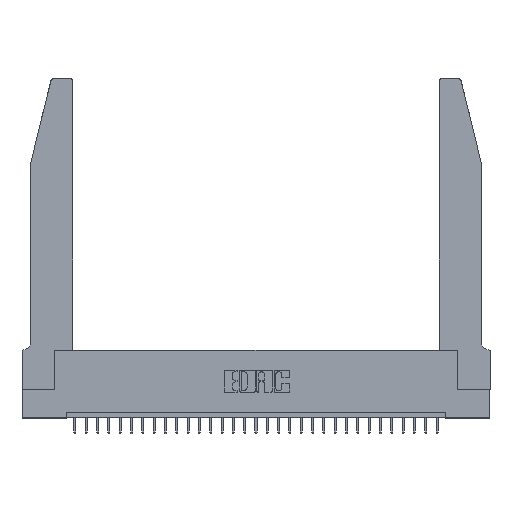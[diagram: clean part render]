
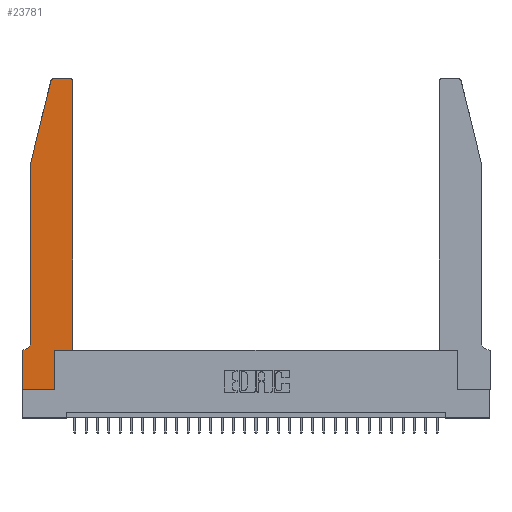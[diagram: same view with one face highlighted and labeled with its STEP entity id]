
A CAD part, top view. The second image highlights one B-rep face of the part: STEP entity #23781.
In plain terms, the highlighted planar face has unit normal (0, 0, 1).
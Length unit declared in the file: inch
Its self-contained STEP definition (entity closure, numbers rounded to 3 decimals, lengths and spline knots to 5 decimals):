
#175 = CARTESIAN_POINT ( 'NONE',  ( 0., 0., 0.37 ) ) ;
#258 = CARTESIAN_POINT ( 'NONE',  ( 0.0055, 0.42, 0.37 ) ) ;
#1079 = VECTOR ( 'NONE', #3744, 39.37008 ) ;
#1533 = VECTOR ( 'NONE', #15672, 39.37008 ) ;
#2079 = EDGE_CURVE ( 'NONE', #27720, #7704, #17153, .T. ) ;
#2528 = CARTESIAN_POINT ( 'NONE',  ( 0.0755, 0.35, 0.37 ) ) ;
#3563 = LINE ( 'NONE', #13246, #11403 ) ;
#3694 = EDGE_CURVE ( 'NONE', #10968, #28322, #28476, .T. ) ;
#3744 = DIRECTION ( 'NONE',  ( -1., 0., 0. ) ) ;
#3778 = LINE ( 'NONE', #15166, #22735 ) ;
#4065 = EDGE_CURVE ( 'NONE', #30191, #10968, #19666, .T. ) ;
#4612 = CARTESIAN_POINT ( 'NONE',  ( 0.2865, 0., 0.37 ) ) ;
#4759 = ORIENTED_EDGE ( 'NONE', *, *, #19439, .T. ) ;
#4913 = CARTESIAN_POINT ( 'NONE',  ( 0.0755, 2., 0.37 ) ) ;
#5375 = DIRECTION ( 'NONE',  ( 1., 0., 0. ) ) ;
#5433 = ORIENTED_EDGE ( 'NONE', *, *, #5878, .T. ) ;
#5679 = AXIS2_PLACEMENT_3D ( 'NONE', #12514, #26454, #17212 ) ;
#5790 = AXIS2_PLACEMENT_3D ( 'NONE', #19240, #7521, #24401 ) ;
#5878 = EDGE_CURVE ( 'NONE', #18002, #7665, #17241, .T. ) ;
#6095 = ORIENTED_EDGE ( 'NONE', *, *, #16498, .T. ) ;
#6484 = ORIENTED_EDGE ( 'NONE', *, *, #21886, .T. ) ;
#7140 = DIRECTION ( 'NONE',  ( 0., 0., -1. ) ) ;
#7355 = VECTOR ( 'NONE', #16372, 39.37008 ) ;
#7521 = DIRECTION ( 'NONE',  ( 0., 0., 1. ) ) ;
#7665 = VERTEX_POINT ( 'NONE', #30874 ) ;
#7704 = VERTEX_POINT ( 'NONE', #16473 ) ;
#8157 = CARTESIAN_POINT ( 'NONE',  ( 0.0055, 0.35, 0.37 ) ) ;
#8969 = ORIENTED_EDGE ( 'NONE', *, *, #2079, .T. ) ;
#9335 = VERTEX_POINT ( 'NONE', #26606 ) ;
#9782 = DIRECTION ( 'NONE',  ( -1., 0., 0. ) ) ;
#10113 = EDGE_CURVE ( 'NONE', #19500, #20860, #25782, .T. ) ;
#10968 = VERTEX_POINT ( 'NONE', #8157 ) ;
#11296 = LINE ( 'NONE', #22716, #1533 ) ;
#11403 = VECTOR ( 'NONE', #22626, 39.37008 ) ;
#11440 = DIRECTION ( 'NONE',  ( -1., 0., 0. ) ) ;
#11490 = ORIENTED_EDGE ( 'NONE', *, *, #20705, .T. ) ;
#11560 = CARTESIAN_POINT ( 'NONE',  ( 0.4505, 0.35, 0.37 ) ) ;
#11625 = ORIENTED_EDGE ( 'NONE', *, *, #3694, .T. ) ;
#11797 = ORIENTED_EDGE ( 'NONE', *, *, #15052, .T. ) ;
#12514 = CARTESIAN_POINT ( 'NONE',  ( 0.4205, 2.72, 0.37 ) ) ;
#12654 = DIRECTION ( 'NONE',  ( 0., 1., 0. ) ) ;
#13246 = CARTESIAN_POINT ( 'NONE',  ( 0., 0., 0.37 ) ) ;
#13286 = DIRECTION ( 'NONE',  ( 0., -1., 0. ) ) ;
#13480 = DIRECTION ( 'NONE',  ( 1., 0., 0. ) ) ;
#14019 = VECTOR ( 'NONE', #28979, 39.37008 ) ;
#14038 = VECTOR ( 'NONE', #13480, 39.37008 ) ;
#14194 = AXIS2_PLACEMENT_3D ( 'NONE', #17400, #17085, #5375 ) ;
#14354 = EDGE_CURVE ( 'NONE', #7704, #9335, #19969, .T. ) ;
#14731 = CARTESIAN_POINT ( 'NONE',  ( 0.4505, 2.72, 0.37 ) ) ;
#15052 = EDGE_CURVE ( 'NONE', #20860, #27720, #11296, .T. ) ;
#15166 = CARTESIAN_POINT ( 'NONE',  ( 0.2865, 0.35, 0.37 ) ) ;
#15672 = DIRECTION ( 'NONE',  ( 0., 1., 0. ) ) ;
#16372 = DIRECTION ( 'NONE',  ( 1., 0., 0. ) ) ;
#16473 = CARTESIAN_POINT ( 'NONE',  ( 0.4205, 2.75, 0.37 ) ) ;
#16498 = EDGE_CURVE ( 'NONE', #27935, #23231, #20816, .T. ) ;
#17085 = DIRECTION ( 'NONE',  ( 0., 0., 1. ) ) ;
#17153 = CIRCLE ( 'NONE', #5679, 0.03 ) ;
#17208 = CARTESIAN_POINT ( 'NONE',  ( 0.25487, 2.72718, 0.37 ) ) ;
#17212 = DIRECTION ( 'NONE',  ( 1., 0., 0. ) ) ;
#17241 = LINE ( 'NONE', #4913, #14019 ) ;
#17400 = CARTESIAN_POINT ( 'NONE',  ( 0.284, 2.72, 0.37 ) ) ;
#18002 = VERTEX_POINT ( 'NONE', #17208 ) ;
#18742 = CARTESIAN_POINT ( 'NONE',  ( 0.0755, 2., 0.37 ) ) ;
#19196 = ORIENTED_EDGE ( 'NONE', *, *, #4065, .T. ) ;
#19240 = CARTESIAN_POINT ( 'NONE',  ( 0., 0.35, 0.37 ) ) ;
#19387 = FACE_OUTER_BOUND ( 'NONE', #22227, .T. ) ;
#19439 = EDGE_CURVE ( 'NONE', #7665, #30191, #21077, .T. ) ;
#19500 = VERTEX_POINT ( 'NONE', #30484 ) ;
#19666 = CIRCLE ( 'NONE', #29685, 0.07 ) ;
#19969 = LINE ( 'NONE', #29538, #1079 ) ;
#20144 = VECTOR ( 'NONE', #13286, 39.37008 ) ;
#20705 = EDGE_CURVE ( 'NONE', #23231, #19500, #3778, .T. ) ;
#20816 = LINE ( 'NONE', #23028, #14038 ) ;
#20860 = VERTEX_POINT ( 'NONE', #11560 ) ;
#21077 = LINE ( 'NONE', #18742, #20144 ) ;
#21381 = CARTESIAN_POINT ( 'NONE',  ( 0., 0.35, 0.37 ) ) ;
#21741 = PLANE ( 'NONE',  #5790 ) ;
#21886 = EDGE_CURVE ( 'NONE', #9335, #18002, #27694, .T. ) ;
#22227 = EDGE_LOOP ( 'NONE', ( #24917, #6484, #5433, #4759, #19196, #11625, #29221, #6095, #11490, #23900, #11797, #8969 ) ) ;
#22626 = DIRECTION ( 'NONE',  ( 0., -1., 0. ) ) ;
#22716 = CARTESIAN_POINT ( 'NONE',  ( 0.4505, 0.35, 0.37 ) ) ;
#22735 = VECTOR ( 'NONE', #12654, 39.37008 ) ;
#23028 = CARTESIAN_POINT ( 'NONE',  ( 0., 0., 0.37 ) ) ;
#23231 = VERTEX_POINT ( 'NONE', #4612 ) ;
#23781 = ADVANCED_FACE ( 'NONE', ( #19387 ), #21741, .T. ) ;
#23900 = ORIENTED_EDGE ( 'NONE', *, *, #10113, .T. ) ;
#24401 = DIRECTION ( 'NONE',  ( 1., 0., 0. ) ) ;
#24626 = CARTESIAN_POINT ( 'NONE',  ( 0.0755, 0.42, 0.37 ) ) ;
#24917 = ORIENTED_EDGE ( 'NONE', *, *, #14354, .T. ) ;
#25464 = CARTESIAN_POINT ( 'NONE',  ( 0.4505, 0.35, 0.37 ) ) ;
#25669 = VECTOR ( 'NONE', #11440, 39.37008 ) ;
#25782 = LINE ( 'NONE', #25464, #7355 ) ;
#26454 = DIRECTION ( 'NONE',  ( 0., 0., 1. ) ) ;
#26606 = CARTESIAN_POINT ( 'NONE',  ( 0.284, 2.75, 0.37 ) ) ;
#27694 = CIRCLE ( 'NONE', #14194, 0.03 ) ;
#27720 = VERTEX_POINT ( 'NONE', #14731 ) ;
#27935 = VERTEX_POINT ( 'NONE', #175 ) ;
#28322 = VERTEX_POINT ( 'NONE', #21381 ) ;
#28476 = LINE ( 'NONE', #2528, #25669 ) ;
#28768 = EDGE_CURVE ( 'NONE', #28322, #27935, #3563, .T. ) ;
#28979 = DIRECTION ( 'NONE',  ( -0.239, -0.971, 0. ) ) ;
#29221 = ORIENTED_EDGE ( 'NONE', *, *, #28768, .T. ) ;
#29538 = CARTESIAN_POINT ( 'NONE',  ( 0.2605, 2.75, 0.37 ) ) ;
#29685 = AXIS2_PLACEMENT_3D ( 'NONE', #258, #7140, #9782 ) ;
#30191 = VERTEX_POINT ( 'NONE', #24626 ) ;
#30484 = CARTESIAN_POINT ( 'NONE',  ( 0.2865, 0.35, 0.37 ) ) ;
#30874 = CARTESIAN_POINT ( 'NONE',  ( 0.0755, 2., 0.37 ) ) ;
